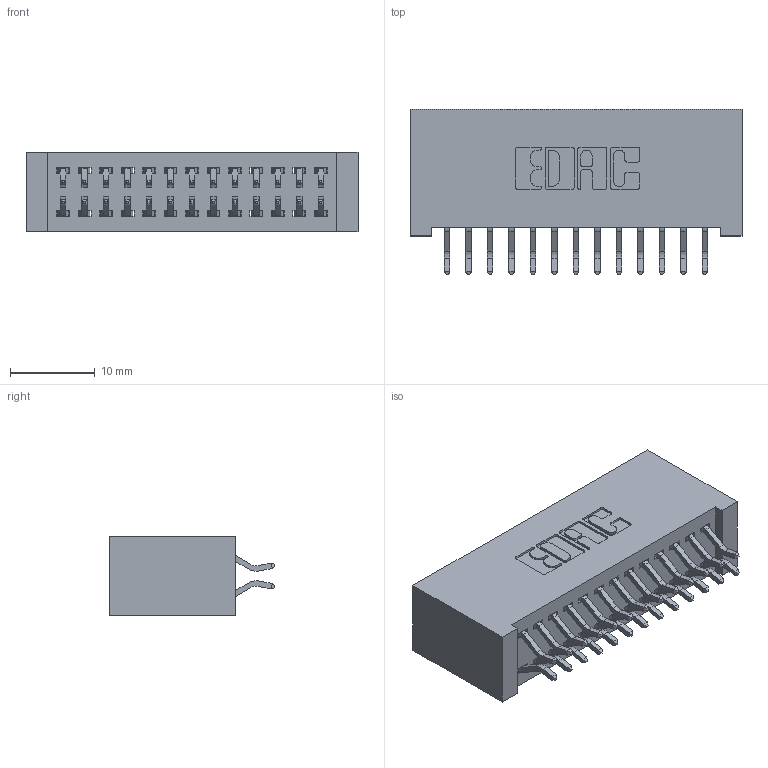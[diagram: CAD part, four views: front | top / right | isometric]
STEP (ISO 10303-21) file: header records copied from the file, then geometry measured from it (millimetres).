
FILE_DESCRIPTION (( 'STEP AP203' ), '1' );
FILE_NAME ('392-026-556-201.STEP', '2019-10-07T11:34:25', ( '' ), ( '' ), 'SwSTEP 2.0', 'SolidWorks 2016', '' );
FILE_SCHEMA (( 'CONFIG_CONTROL_DESIGN' ));
Length unit declared in the file: inch
Products named in the file (3): 342 Part_Lugless; 345-292-001_556 Tail; 392-026-556-201
Assembly tree (27 placements, depth 2):
  392-026-556-201
    342 Part_Lugless
    345-292-001_556 Tail  x26
Bounding box: 39.27 x 19.58 x 9.4 mm (x, y, z)
Volume: 3829.8 mm3; surface area: 5940.5 mm2
Topology: 27 solids, 27 shells, 1610 faces, 4773 edges, 3146 vertices
Faces by surface type: plane 1102, cylinder 508
Entity records: 11925 total; most frequent: CARTESIAN_POINT 2022, ORIENTED_EDGE 1946, DIRECTION 1761, EDGE_CURVE 973, LINE 845, VECTOR 845, VERTEX_POINT 646, AXIS2_PLACEMENT_3D 458
